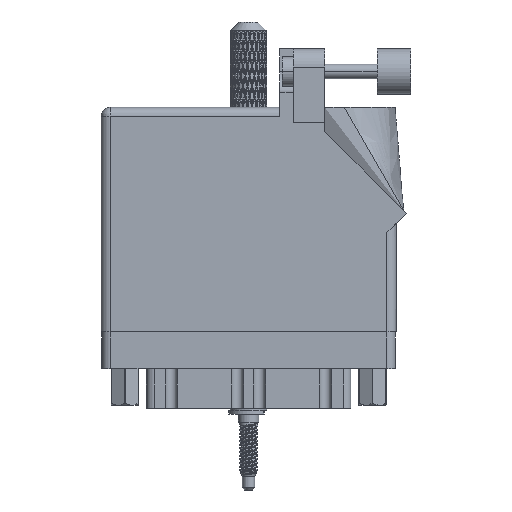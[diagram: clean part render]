
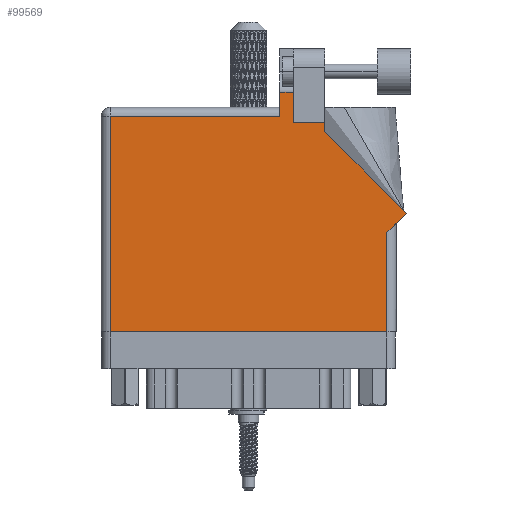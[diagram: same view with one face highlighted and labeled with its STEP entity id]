
A CAD part, front view. The second image highlights one B-rep face of the part: STEP entity #99569.
In plain terms, the highlighted face is planar.
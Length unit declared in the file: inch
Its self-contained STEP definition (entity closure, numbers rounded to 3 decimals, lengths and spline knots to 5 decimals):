
#1035 = EDGE_CURVE ( 'NONE', #24715, #73995, #29375, .T. ) ;
#2140 = CARTESIAN_POINT ( 'NONE',  ( 1.948, 0.737, 0. ) ) ;
#4595 = VECTOR ( 'NONE', #56546, 39.37008 ) ;
#8163 = VERTEX_POINT ( 'NONE', #70012 ) ;
#10396 = EDGE_LOOP ( 'NONE', ( #26786, #14041, #97801, #20552, #80084, #49844, #51276, #75835, #105238, #39924, #50412 ) ) ;
#10535 = VERTEX_POINT ( 'NONE', #75482 ) ;
#11929 = VERTEX_POINT ( 'NONE', #53609 ) ;
#12452 = EDGE_CURVE ( 'NONE', #22989, #8163, #23548, .T. ) ;
#12647 = CARTESIAN_POINT ( 'NONE',  ( 2.08071, 0.80771, 0. ) ) ;
#13566 = PLANE ( 'NONE',  #92273 ) ;
#13979 = VERTEX_POINT ( 'NONE', #18913 ) ;
#14041 = ORIENTED_EDGE ( 'NONE', *, *, #12452, .T. ) ;
#14436 = VECTOR ( 'NONE', #76785, 39.37008 ) ;
#15154 = DIRECTION ( 'NONE',  ( 0., -1., 0. ) ) ;
#16715 = VECTOR ( 'NONE', #36859, 39.37008 ) ;
#18656 = EDGE_CURVE ( 'NONE', #63119, #11929, #73772, .T. ) ;
#18913 = CARTESIAN_POINT ( 'NONE',  ( 1.948, 0.675, 0. ) ) ;
#19631 = CARTESIAN_POINT ( 'NONE',  ( 0.062, 0., 0. ) ) ;
#20552 = ORIENTED_EDGE ( 'NONE', *, *, #1035, .T. ) ;
#21873 = CARTESIAN_POINT ( 'NONE',  ( 0., 1.468, 0. ) ) ;
#22989 = VERTEX_POINT ( 'NONE', #44455 ) ;
#23548 = LINE ( 'NONE', #67742, #113358 ) ;
#24715 = VERTEX_POINT ( 'NONE', #67711 ) ;
#25503 = DIRECTION ( 'NONE',  ( 0., 1., 0. ) ) ;
#25672 = LINE ( 'NONE', #34833, #14436 ) ;
#26786 = ORIENTED_EDGE ( 'NONE', *, *, #77808, .T. ) ;
#29375 = LINE ( 'NONE', #21873, #43130 ) ;
#33382 = VECTOR ( 'NONE', #105392, 39.37008 ) ;
#34833 = CARTESIAN_POINT ( 'NONE',  ( 2.08071, 0.80771, 0. ) ) ;
#36859 = DIRECTION ( 'NONE',  ( 0., -1., 0. ) ) ;
#37208 = DIRECTION ( 'NONE',  ( 0., 1., 0. ) ) ;
#38836 = CARTESIAN_POINT ( 'NONE',  ( 0.062, 1.468, 0. ) ) ;
#39596 = EDGE_CURVE ( 'NONE', #10535, #13979, #80267, .T. ) ;
#39924 = ORIENTED_EDGE ( 'NONE', *, *, #60088, .T. ) ;
#43130 = VECTOR ( 'NONE', #111824, 39.37008 ) ;
#44455 = CARTESIAN_POINT ( 'NONE',  ( 1.311, 1.6315, 0. ) ) ;
#46326 = EDGE_CURVE ( 'NONE', #73995, #91747, #86432, .T. ) ;
#49844 = ORIENTED_EDGE ( 'NONE', *, *, #76141, .T. ) ;
#50412 = ORIENTED_EDGE ( 'NONE', *, *, #18656, .T. ) ;
#51276 = ORIENTED_EDGE ( 'NONE', *, *, #39596, .T. ) ;
#53609 = CARTESIAN_POINT ( 'NONE',  ( 1.311, 1.43, 0. ) ) ;
#54734 = CARTESIAN_POINT ( 'NONE',  ( 1.524, 1.43, 0. ) ) ;
#54819 = LINE ( 'NONE', #90947, #86189 ) ;
#56384 = CARTESIAN_POINT ( 'NONE',  ( 0.062, 0., 0. ) ) ;
#56546 = DIRECTION ( 'NONE',  ( -1., 0., 0. ) ) ;
#56644 = CARTESIAN_POINT ( 'NONE',  ( 0., 1.53, 0. ) ) ;
#60088 = EDGE_CURVE ( 'NONE', #104189, #63119, #86350, .T. ) ;
#63119 = VERTEX_POINT ( 'NONE', #54734 ) ;
#63574 = EDGE_CURVE ( 'NONE', #113474, #104189, #25672, .T. ) ;
#66276 = CARTESIAN_POINT ( 'NONE',  ( 1.524, 1.43, 0. ) ) ;
#67711 = CARTESIAN_POINT ( 'NONE',  ( 1.217, 1.468, 0. ) ) ;
#67742 = CARTESIAN_POINT ( 'NONE',  ( 1.64177, 1.6315, 0. ) ) ;
#68706 = LINE ( 'NONE', #112887, #33382 ) ;
#70012 = CARTESIAN_POINT ( 'NONE',  ( 1.217, 1.6315, 0. ) ) ;
#71062 = CARTESIAN_POINT ( 'NONE',  ( 1.311, 1.43, 0. ) ) ;
#72258 = VECTOR ( 'NONE', #37208, 39.37008 ) ;
#72770 = LINE ( 'NONE', #71062, #99579 ) ;
#72810 = VECTOR ( 'NONE', #25503, 39.37008 ) ;
#73772 = LINE ( 'NONE', #66276, #4595 ) ;
#73995 = VERTEX_POINT ( 'NONE', #38836 ) ;
#75346 = CARTESIAN_POINT ( 'NONE',  ( 1.524, 1.36442, 0. ) ) ;
#75482 = CARTESIAN_POINT ( 'NONE',  ( 1.948, 0., 0. ) ) ;
#75835 = ORIENTED_EDGE ( 'NONE', *, *, #111502, .T. ) ;
#76030 = CARTESIAN_POINT ( 'NONE',  ( 1.217, 1.53, 0. ) ) ;
#76141 = EDGE_CURVE ( 'NONE', #91747, #10535, #68706, .T. ) ;
#76785 = DIRECTION ( 'NONE',  ( -0.707, 0.707, 0. ) ) ;
#77808 = EDGE_CURVE ( 'NONE', #11929, #22989, #72770, .T. ) ;
#80084 = ORIENTED_EDGE ( 'NONE', *, *, #46326, .T. ) ;
#80267 = LINE ( 'NONE', #2140, #72258 ) ;
#83481 = DIRECTION ( 'NONE',  ( 0.707, 0.707, 0. ) ) ;
#83498 = LINE ( 'NONE', #76030, #84921 ) ;
#84921 = VECTOR ( 'NONE', #15154, 39.37008 ) ;
#86189 = VECTOR ( 'NONE', #83481, 39.37008 ) ;
#86350 = LINE ( 'NONE', #94389, #72810 ) ;
#86432 = LINE ( 'NONE', #19631, #16715 ) ;
#90947 = CARTESIAN_POINT ( 'NONE',  ( 2.01, 0.737, 0. ) ) ;
#91635 = DIRECTION ( 'NONE',  ( 0., 0., -1. ) ) ;
#91747 = VERTEX_POINT ( 'NONE', #56384 ) ;
#92273 = AXIS2_PLACEMENT_3D ( 'NONE', #56644, #91635, #108289 ) ;
#94389 = CARTESIAN_POINT ( 'NONE',  ( 1.524, 1.36442, 0. ) ) ;
#97444 = DIRECTION ( 'NONE',  ( 0., 1., 0. ) ) ;
#97801 = ORIENTED_EDGE ( 'NONE', *, *, #102043, .T. ) ;
#99129 = FACE_OUTER_BOUND ( 'NONE', #10396, .T. ) ;
#99569 = ADVANCED_FACE ( 'NONE', ( #99129 ), #13566, .F. ) ;
#99579 = VECTOR ( 'NONE', #97444, 39.37008 ) ;
#100471 = DIRECTION ( 'NONE',  ( -1., 0., 0. ) ) ;
#102043 = EDGE_CURVE ( 'NONE', #8163, #24715, #83498, .T. ) ;
#104189 = VERTEX_POINT ( 'NONE', #75346 ) ;
#105238 = ORIENTED_EDGE ( 'NONE', *, *, #63574, .T. ) ;
#105392 = DIRECTION ( 'NONE',  ( 1., 0., 0. ) ) ;
#108289 = DIRECTION ( 'NONE',  ( -1., 0., 0. ) ) ;
#111502 = EDGE_CURVE ( 'NONE', #13979, #113474, #54819, .T. ) ;
#111824 = DIRECTION ( 'NONE',  ( -1., 0., 0. ) ) ;
#112887 = CARTESIAN_POINT ( 'NONE',  ( 0., 0., 0. ) ) ;
#113358 = VECTOR ( 'NONE', #100471, 39.37008 ) ;
#113474 = VERTEX_POINT ( 'NONE', #12647 ) ;
